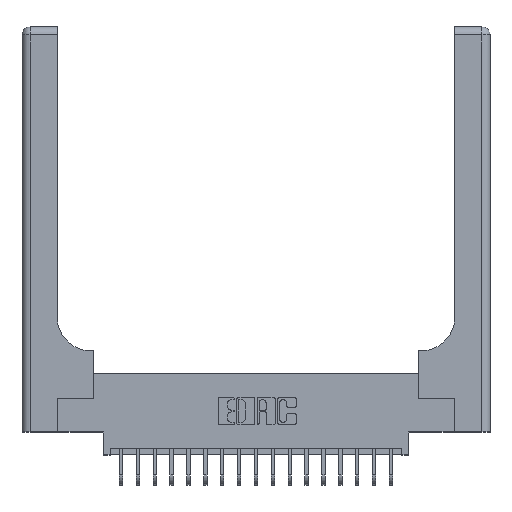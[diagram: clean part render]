
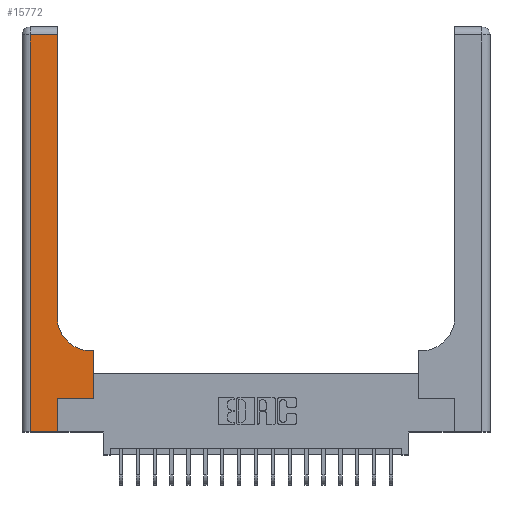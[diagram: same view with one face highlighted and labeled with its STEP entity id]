
A CAD part, top view. The second image highlights one B-rep face of the part: STEP entity #15772.
In plain terms, the highlighted planar face has unit normal (0, 0, 1).
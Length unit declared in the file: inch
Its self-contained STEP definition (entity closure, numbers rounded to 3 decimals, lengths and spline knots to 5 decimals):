
#584 = CARTESIAN_POINT ( 'NONE',  ( 0.528, 0.25, 0.37 ) ) ;
#655 = VECTOR ( 'NONE', #17047, 39.37008 ) ;
#1214 = EDGE_CURVE ( 'NONE', #18816, #13148, #14737, .T. ) ;
#1312 = ORIENTED_EDGE ( 'NONE', *, *, #20125, .T. ) ;
#1423 = CARTESIAN_POINT ( 'NONE',  ( 0.26, 2.94, 0.37 ) ) ;
#2564 = CARTESIAN_POINT ( 'NONE',  ( 0.265, 0., 0.37 ) ) ;
#3962 = CARTESIAN_POINT ( 'NONE',  ( 0.26, 0.6, 0.37 ) ) ;
#4046 = LINE ( 'NONE', #584, #17721 ) ;
#4169 = CARTESIAN_POINT ( 'NONE',  ( 0.51, 0.6, 0.37 ) ) ;
#4279 = AXIS2_PLACEMENT_3D ( 'NONE', #21411, #4607, #11392 ) ;
#4501 = CARTESIAN_POINT ( 'NONE',  ( 0.265, 0.25, 0.37 ) ) ;
#4517 = CARTESIAN_POINT ( 'NONE',  ( 0., 3., 0.37 ) ) ;
#4607 = DIRECTION ( 'NONE',  ( 0., 0., -1. ) ) ;
#4927 = LINE ( 'NONE', #18607, #655 ) ;
#4956 = LINE ( 'NONE', #8393, #12752 ) ;
#5070 = DIRECTION ( 'NONE',  ( 0., 1., 0. ) ) ;
#5099 = ORIENTED_EDGE ( 'NONE', *, *, #16196, .T. ) ;
#6013 = CARTESIAN_POINT ( 'NONE',  ( 0., 2.94, 0.37 ) ) ;
#6600 = CARTESIAN_POINT ( 'NONE',  ( 0.06, 3., 0.37 ) ) ;
#6998 = ORIENTED_EDGE ( 'NONE', *, *, #14292, .T. ) ;
#7984 = DIRECTION ( 'NONE',  ( -1., 0., 0. ) ) ;
#8393 = CARTESIAN_POINT ( 'NONE',  ( 0.265, 0., 0.37 ) ) ;
#8453 = VERTEX_POINT ( 'NONE', #1423 ) ;
#8478 = VECTOR ( 'NONE', #9067, 39.37008 ) ;
#8543 = AXIS2_PLACEMENT_3D ( 'NONE', #4517, #11417, #7984 ) ;
#9030 = ORIENTED_EDGE ( 'NONE', *, *, #13153, .T. ) ;
#9067 = DIRECTION ( 'NONE',  ( -1., 0., 0. ) ) ;
#9094 = VERTEX_POINT ( 'NONE', #17953 ) ;
#9191 = CARTESIAN_POINT ( 'NONE',  ( 0.528, 0.25, 0.37 ) ) ;
#9262 = EDGE_CURVE ( 'NONE', #9094, #18816, #13492, .T. ) ;
#9349 = LINE ( 'NONE', #6013, #12360 ) ;
#9402 = CARTESIAN_POINT ( 'NONE',  ( 0.528, 0.6, 0.37 ) ) ;
#9471 = VECTOR ( 'NONE', #13165, 39.37008 ) ;
#9692 = EDGE_LOOP ( 'NONE', ( #11884, #9030, #16001, #16008, #21300, #6998, #1312, #9778, #5099 ) ) ;
#9778 = ORIENTED_EDGE ( 'NONE', *, *, #12085, .T. ) ;
#10275 = VECTOR ( 'NONE', #19214, 39.37008 ) ;
#10300 = VERTEX_POINT ( 'NONE', #4169 ) ;
#10378 = VECTOR ( 'NONE', #14516, 39.37008 ) ;
#11392 = DIRECTION ( 'NONE',  ( 1., 0., 0. ) ) ;
#11417 = DIRECTION ( 'NONE',  ( 0., 0., -1. ) ) ;
#11884 = ORIENTED_EDGE ( 'NONE', *, *, #21483, .T. ) ;
#12085 = EDGE_CURVE ( 'NONE', #17379, #10300, #17526, .T. ) ;
#12163 = DIRECTION ( 'NONE',  ( 0., 1., 0. ) ) ;
#12221 = VERTEX_POINT ( 'NONE', #4501 ) ;
#12239 = CARTESIAN_POINT ( 'NONE',  ( 0.26, 0.85, 0.37 ) ) ;
#12360 = VECTOR ( 'NONE', #17908, 39.37008 ) ;
#12682 = CARTESIAN_POINT ( 'NONE',  ( 0.06, 0., 0.37 ) ) ;
#12752 = VECTOR ( 'NONE', #5070, 39.37008 ) ;
#13148 = VERTEX_POINT ( 'NONE', #2564 ) ;
#13153 = EDGE_CURVE ( 'NONE', #8453, #9094, #9349, .T. ) ;
#13165 = DIRECTION ( 'NONE',  ( 0., -1., 0. ) ) ;
#13492 = LINE ( 'NONE', #6600, #9471 ) ;
#13859 = CIRCLE ( 'NONE', #4279, 0.25 ) ;
#14292 = EDGE_CURVE ( 'NONE', #12221, #19687, #15758, .T. ) ;
#14516 = DIRECTION ( 'NONE',  ( 1., 0., 0. ) ) ;
#14617 = EDGE_CURVE ( 'NONE', #13148, #12221, #4956, .T. ) ;
#14737 = LINE ( 'NONE', #16199, #10378 ) ;
#15758 = LINE ( 'NONE', #17870, #10275 ) ;
#15772 = ADVANCED_FACE ( 'NONE', ( #16635 ), #16530, .F. ) ;
#16001 = ORIENTED_EDGE ( 'NONE', *, *, #9262, .T. ) ;
#16008 = ORIENTED_EDGE ( 'NONE', *, *, #1214, .T. ) ;
#16196 = EDGE_CURVE ( 'NONE', #10300, #18677, #13859, .T. ) ;
#16199 = CARTESIAN_POINT ( 'NONE',  ( 0., 0., 0.37 ) ) ;
#16530 = PLANE ( 'NONE',  #8543 ) ;
#16635 = FACE_OUTER_BOUND ( 'NONE', #9692, .T. ) ;
#17047 = DIRECTION ( 'NONE',  ( 0., 1., 0. ) ) ;
#17379 = VERTEX_POINT ( 'NONE', #9402 ) ;
#17526 = LINE ( 'NONE', #3962, #8478 ) ;
#17721 = VECTOR ( 'NONE', #12163, 39.37008 ) ;
#17870 = CARTESIAN_POINT ( 'NONE',  ( 0.265, 0.25, 0.37 ) ) ;
#17908 = DIRECTION ( 'NONE',  ( -1., 0., 0. ) ) ;
#17953 = CARTESIAN_POINT ( 'NONE',  ( 0.06, 2.94, 0.37 ) ) ;
#18607 = CARTESIAN_POINT ( 'NONE',  ( 0.26, 3., 0.37 ) ) ;
#18677 = VERTEX_POINT ( 'NONE', #12239 ) ;
#18816 = VERTEX_POINT ( 'NONE', #12682 ) ;
#19214 = DIRECTION ( 'NONE',  ( 1., 0., 0. ) ) ;
#19687 = VERTEX_POINT ( 'NONE', #9191 ) ;
#20125 = EDGE_CURVE ( 'NONE', #19687, #17379, #4046, .T. ) ;
#21300 = ORIENTED_EDGE ( 'NONE', *, *, #14617, .T. ) ;
#21411 = CARTESIAN_POINT ( 'NONE',  ( 0.51, 0.85, 0.37 ) ) ;
#21483 = EDGE_CURVE ( 'NONE', #18677, #8453, #4927, .T. ) ;
